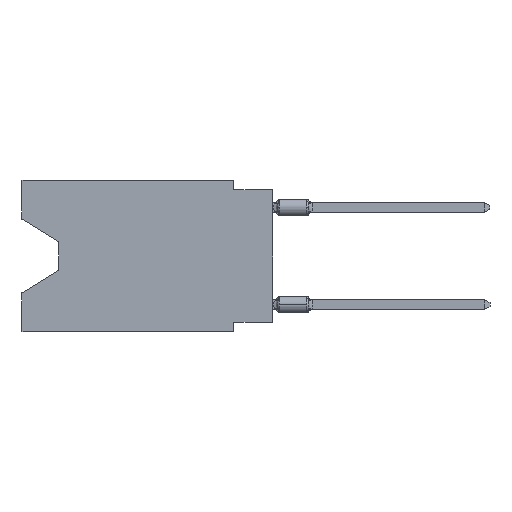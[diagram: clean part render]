
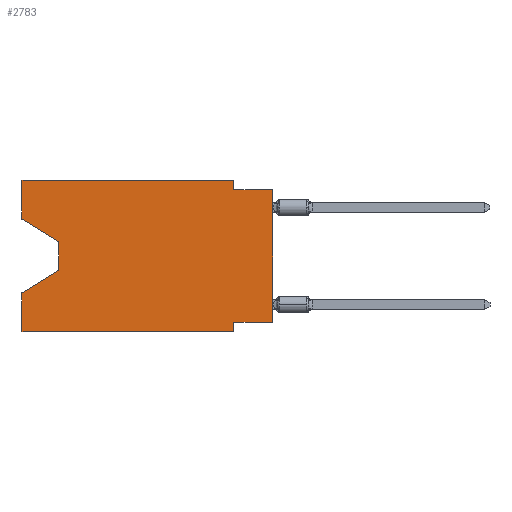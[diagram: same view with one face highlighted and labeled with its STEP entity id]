
A CAD part, left-side view. The second image highlights one B-rep face of the part: STEP entity #2783.
In plain terms, the highlighted planar face has unit normal (-1, 0, 0).
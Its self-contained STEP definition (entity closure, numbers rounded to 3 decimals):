
#8 = EDGE_CURVE ( 'NONE', #3927, #6335, #13562, .T. ) ;
#110 = ORIENTED_EDGE ( 'NONE', *, *, #17794, .F. ) ;
#430 = DIRECTION ( 'NONE',  ( 0., 0., -1. ) ) ;
#497 = CARTESIAN_POINT ( 'NONE',  ( 0., 13.97, -4.013 ) ) ;
#553 = VECTOR ( 'NONE', #2595, 1000. ) ;
#666 = CARTESIAN_POINT ( 'NONE',  ( 0., 2.54, -9.906 ) ) ;
#670 = CARTESIAN_POINT ( 'NONE',  ( 0., 2.54, 0. ) ) ;
#825 = CARTESIAN_POINT ( 'NONE',  ( 0., 2.54, -0.635 ) ) ;
#981 = EDGE_CURVE ( 'NONE', #3203, #12871, #8752, .T. ) ;
#1166 = EDGE_CURVE ( 'NONE', #20536, #11851, #16253, .T. ) ;
#1395 = VERTEX_POINT ( 'NONE', #13710 ) ;
#1401 = EDGE_LOOP ( 'NONE', ( #18418, #21498, #3089, #16211, #14385, #110, #4946, #18076, #19295, #22591, #8611, #10950 ) ) ;
#2175 = CARTESIAN_POINT ( 'NONE',  ( 0., 0., -0.635 ) ) ;
#2370 = VECTOR ( 'NONE', #3886, 1000. ) ;
#2509 = DIRECTION ( 'NONE',  ( 0., 0., 1. ) ) ;
#2595 = DIRECTION ( 'NONE',  ( 0., 0., 1. ) ) ;
#2783 = ADVANCED_FACE ( 'NONE', ( #12434 ), #9285, .F. ) ;
#2912 = CARTESIAN_POINT ( 'NONE',  ( 0., 16.383, 0. ) ) ;
#3073 = CARTESIAN_POINT ( 'NONE',  ( 0., 16.383, -7.36 ) ) ;
#3089 = ORIENTED_EDGE ( 'NONE', *, *, #981, .T. ) ;
#3203 = VERTEX_POINT ( 'NONE', #3729 ) ;
#3216 = CARTESIAN_POINT ( 'NONE',  ( 0., 16.383, 0. ) ) ;
#3611 = VECTOR ( 'NONE', #8158, 1000. ) ;
#3729 = CARTESIAN_POINT ( 'NONE',  ( 0., 13.97, -5.893 ) ) ;
#3833 = LINE ( 'NONE', #16196, #12020 ) ;
#3886 = DIRECTION ( 'NONE',  ( 0., 1., 0. ) ) ;
#3927 = VERTEX_POINT ( 'NONE', #15561 ) ;
#3998 = LINE ( 'NONE', #666, #6536 ) ;
#4224 = LINE ( 'NONE', #11274, #7696 ) ;
#4375 = LINE ( 'NONE', #18009, #8942 ) ;
#4763 = EDGE_CURVE ( 'NONE', #13641, #8888, #4375, .T. ) ;
#4899 = LINE ( 'NONE', #6658, #3611 ) ;
#4946 = ORIENTED_EDGE ( 'NONE', *, *, #1166, .F. ) ;
#5139 = CARTESIAN_POINT ( 'NONE',  ( 0., 16.383, -9.906 ) ) ;
#5238 = VERTEX_POINT ( 'NONE', #670 ) ;
#5620 = CARTESIAN_POINT ( 'NONE',  ( 0., 0., -9.271 ) ) ;
#6335 = VERTEX_POINT ( 'NONE', #3216 ) ;
#6536 = VECTOR ( 'NONE', #13126, 1000. ) ;
#6658 = CARTESIAN_POINT ( 'NONE',  ( 0., 16.383, 0. ) ) ;
#6677 = CARTESIAN_POINT ( 'NONE',  ( 0., 2.54, -9.271 ) ) ;
#7414 = DIRECTION ( 'NONE',  ( 0., 0., -1. ) ) ;
#7603 = VECTOR ( 'NONE', #21716, 1000. ) ;
#7637 = LINE ( 'NONE', #14682, #7603 ) ;
#7696 = VECTOR ( 'NONE', #2509, 1000. ) ;
#7993 = LINE ( 'NONE', #2912, #12730 ) ;
#8158 = DIRECTION ( 'NONE',  ( 0., -1., 0. ) ) ;
#8611 = ORIENTED_EDGE ( 'NONE', *, *, #19068, .F. ) ;
#8752 = LINE ( 'NONE', #22608, #19679 ) ;
#8888 = VERTEX_POINT ( 'NONE', #2175 ) ;
#8942 = VECTOR ( 'NONE', #16385, 1000. ) ;
#9017 = DIRECTION ( 'NONE',  ( 0., 0., -1. ) ) ;
#9102 = VERTEX_POINT ( 'NONE', #5139 ) ;
#9285 = PLANE ( 'NONE',  #17534 ) ;
#10174 = VECTOR ( 'NONE', #15150, 1000. ) ;
#10791 = DIRECTION ( 'NONE',  ( 1., 0., 0. ) ) ;
#10862 = VERTEX_POINT ( 'NONE', #16426 ) ;
#10950 = ORIENTED_EDGE ( 'NONE', *, *, #8, .F. ) ;
#11274 = CARTESIAN_POINT ( 'NONE',  ( 0., 0., 0. ) ) ;
#11667 = VECTOR ( 'NONE', #9017, 1000. ) ;
#11851 = VERTEX_POINT ( 'NONE', #6677 ) ;
#12020 = VECTOR ( 'NONE', #7414, 1000. ) ;
#12434 = FACE_OUTER_BOUND ( 'NONE', #1401, .T. ) ;
#12730 = VECTOR ( 'NONE', #15385, 1000. ) ;
#12871 = VERTEX_POINT ( 'NONE', #3073 ) ;
#13058 = LINE ( 'NONE', #19868, #10174 ) ;
#13126 = DIRECTION ( 'NONE',  ( 0., 0., -1. ) ) ;
#13154 = EDGE_CURVE ( 'NONE', #9102, #12871, #7993, .T. ) ;
#13562 = LINE ( 'NONE', #20596, #553 ) ;
#13641 = VERTEX_POINT ( 'NONE', #825 ) ;
#13710 = CARTESIAN_POINT ( 'NONE',  ( 0., 2.54, -9.906 ) ) ;
#13846 = DIRECTION ( 'NONE',  ( 0., 0.855, -0.519 ) ) ;
#14385 = ORIENTED_EDGE ( 'NONE', *, *, #15971, .T. ) ;
#14682 = CARTESIAN_POINT ( 'NONE',  ( 0., 16.383, -9.906 ) ) ;
#15150 = DIRECTION ( 'NONE',  ( 0., -0.855, -0.519 ) ) ;
#15385 = DIRECTION ( 'NONE',  ( 0., 0., 1. ) ) ;
#15561 = CARTESIAN_POINT ( 'NONE',  ( 0., 16.383, -2.546 ) ) ;
#15569 = EDGE_CURVE ( 'NONE', #5238, #13641, #3833, .T. ) ;
#15794 = EDGE_CURVE ( 'NONE', #10862, #3203, #17691, .T. ) ;
#15952 = EDGE_CURVE ( 'NONE', #3927, #10862, #13058, .T. ) ;
#15971 = EDGE_CURVE ( 'NONE', #9102, #1395, #7637, .T. ) ;
#16196 = CARTESIAN_POINT ( 'NONE',  ( 0., 2.54, 0. ) ) ;
#16211 = ORIENTED_EDGE ( 'NONE', *, *, #13154, .F. ) ;
#16253 = LINE ( 'NONE', #5620, #2370 ) ;
#16385 = DIRECTION ( 'NONE',  ( 0., -1., 0. ) ) ;
#16426 = CARTESIAN_POINT ( 'NONE',  ( 0., 13.97, -4.013 ) ) ;
#17467 = CARTESIAN_POINT ( 'NONE',  ( 0., 0., -9.271 ) ) ;
#17534 = AXIS2_PLACEMENT_3D ( 'NONE', #19571, #10791, #430 ) ;
#17691 = LINE ( 'NONE', #497, #11667 ) ;
#17794 = EDGE_CURVE ( 'NONE', #11851, #1395, #3998, .T. ) ;
#18009 = CARTESIAN_POINT ( 'NONE',  ( 0., 0., -0.635 ) ) ;
#18076 = ORIENTED_EDGE ( 'NONE', *, *, #18987, .T. ) ;
#18418 = ORIENTED_EDGE ( 'NONE', *, *, #15952, .T. ) ;
#18987 = EDGE_CURVE ( 'NONE', #20536, #8888, #4224, .T. ) ;
#19068 = EDGE_CURVE ( 'NONE', #6335, #5238, #4899, .T. ) ;
#19295 = ORIENTED_EDGE ( 'NONE', *, *, #4763, .F. ) ;
#19571 = CARTESIAN_POINT ( 'NONE',  ( 0., 16.383, 0. ) ) ;
#19679 = VECTOR ( 'NONE', #13846, 1000. ) ;
#19868 = CARTESIAN_POINT ( 'NONE',  ( 0., 16.383, -2.546 ) ) ;
#20536 = VERTEX_POINT ( 'NONE', #17467 ) ;
#20596 = CARTESIAN_POINT ( 'NONE',  ( 0., 16.383, 0. ) ) ;
#21498 = ORIENTED_EDGE ( 'NONE', *, *, #15794, .T. ) ;
#21716 = DIRECTION ( 'NONE',  ( 0., -1., 0. ) ) ;
#22591 = ORIENTED_EDGE ( 'NONE', *, *, #15569, .F. ) ;
#22608 = CARTESIAN_POINT ( 'NONE',  ( 0., 13.97, -5.893 ) ) ;
